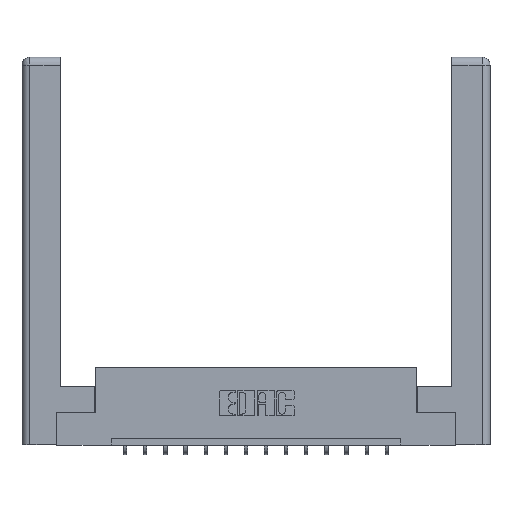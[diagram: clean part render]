
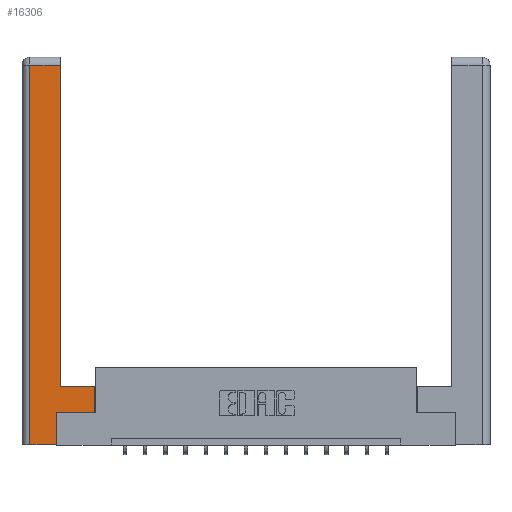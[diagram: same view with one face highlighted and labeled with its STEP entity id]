
A CAD part, top view. The second image highlights one B-rep face of the part: STEP entity #16306.
In plain terms, the highlighted planar face has unit normal (0, 0, 1).
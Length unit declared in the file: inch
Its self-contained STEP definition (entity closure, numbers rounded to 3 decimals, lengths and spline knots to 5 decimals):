
#33 = VECTOR ( 'NONE', #9233, 39.37008 ) ;
#392 = VERTEX_POINT ( 'NONE', #15237 ) ;
#905 = CARTESIAN_POINT ( 'NONE',  ( 0.265, 0.245, 0. ) ) ;
#1146 = LINE ( 'NONE', #4113, #2574 ) ;
#1527 = VERTEX_POINT ( 'NONE', #14548 ) ;
#2090 = CARTESIAN_POINT ( 'NONE',  ( 0.0615, 2.94, 0. ) ) ;
#2414 = CARTESIAN_POINT ( 'NONE',  ( 0.565, 0.45, 0. ) ) ;
#2574 = VECTOR ( 'NONE', #15525, 39.37008 ) ;
#2589 = DIRECTION ( 'NONE',  ( -1., 0., 0. ) ) ;
#2604 = VECTOR ( 'NONE', #15812, 39.37008 ) ;
#2819 = ORIENTED_EDGE ( 'NONE', *, *, #16593, .T. ) ;
#3337 = CARTESIAN_POINT ( 'NONE',  ( 0.565, 0.45, 0. ) ) ;
#3830 = CARTESIAN_POINT ( 'NONE',  ( 0.565, 0.245, 0. ) ) ;
#3939 = DIRECTION ( 'NONE',  ( 1., 0., 0. ) ) ;
#4113 = CARTESIAN_POINT ( 'NONE',  ( 0.0615, 0., 0. ) ) ;
#4242 = CARTESIAN_POINT ( 'NONE',  ( 0.295, 3., 0. ) ) ;
#4461 = VERTEX_POINT ( 'NONE', #2090 ) ;
#4954 = VERTEX_POINT ( 'NONE', #13123 ) ;
#5233 = LINE ( 'NONE', #2414, #7033 ) ;
#5357 = VECTOR ( 'NONE', #7497, 39.37008 ) ;
#5381 = EDGE_CURVE ( 'NONE', #392, #14275, #13060, .T. ) ;
#6147 = EDGE_CURVE ( 'NONE', #7818, #11671, #10586, .T. ) ;
#6274 = CARTESIAN_POINT ( 'NONE',  ( 0.295, 0.45, 0. ) ) ;
#6314 = CARTESIAN_POINT ( 'NONE',  ( 0.0615, 2.94, 0. ) ) ;
#6333 = DIRECTION ( 'NONE',  ( 0., 1., 0. ) ) ;
#7033 = VECTOR ( 'NONE', #6333, 39.37008 ) ;
#7497 = DIRECTION ( 'NONE',  ( 0., 1., 0. ) ) ;
#7818 = VERTEX_POINT ( 'NONE', #3337 ) ;
#8476 = LINE ( 'NONE', #15450, #15582 ) ;
#9026 = DIRECTION ( 'NONE',  ( 0., 0., -1. ) ) ;
#9233 = DIRECTION ( 'NONE',  ( -1., 0., 0. ) ) ;
#9713 = CARTESIAN_POINT ( 'NONE',  ( 0.265, 0., 0. ) ) ;
#9742 = ORIENTED_EDGE ( 'NONE', *, *, #6147, .T. ) ;
#9832 = LINE ( 'NONE', #9713, #12288 ) ;
#9867 = ORIENTED_EDGE ( 'NONE', *, *, #14572, .T. ) ;
#10187 = VECTOR ( 'NONE', #10888, 39.37008 ) ;
#10586 = LINE ( 'NONE', #15915, #33 ) ;
#10695 = EDGE_CURVE ( 'NONE', #4954, #4461, #14246, .T. ) ;
#10888 = DIRECTION ( 'NONE',  ( -1., 0., 0. ) ) ;
#11099 = FACE_OUTER_BOUND ( 'NONE', #14337, .T. ) ;
#11671 = VERTEX_POINT ( 'NONE', #6274 ) ;
#11720 = DIRECTION ( 'NONE',  ( 1., 0., 0. ) ) ;
#12142 = ORIENTED_EDGE ( 'NONE', *, *, #16000, .T. ) ;
#12288 = VECTOR ( 'NONE', #11720, 39.37008 ) ;
#12792 = VERTEX_POINT ( 'NONE', #3830 ) ;
#12911 = PLANE ( 'NONE',  #12947 ) ;
#12947 = AXIS2_PLACEMENT_3D ( 'NONE', #16766, #9026, #2589 ) ;
#12950 = LINE ( 'NONE', #4242, #2604 ) ;
#13060 = LINE ( 'NONE', #905, #5357 ) ;
#13123 = CARTESIAN_POINT ( 'NONE',  ( 0.295, 2.94, 0. ) ) ;
#13179 = EDGE_CURVE ( 'NONE', #14275, #12792, #8476, .T. ) ;
#13532 = ORIENTED_EDGE ( 'NONE', *, *, #13179, .T. ) ;
#13865 = EDGE_CURVE ( 'NONE', #12792, #7818, #5233, .T. ) ;
#14082 = ORIENTED_EDGE ( 'NONE', *, *, #10695, .T. ) ;
#14246 = LINE ( 'NONE', #6314, #10187 ) ;
#14275 = VERTEX_POINT ( 'NONE', #14389 ) ;
#14337 = EDGE_LOOP ( 'NONE', ( #12142, #14082, #2819, #9867, #14625, #13532, #15276, #9742 ) ) ;
#14389 = CARTESIAN_POINT ( 'NONE',  ( 0.265, 0.245, 0. ) ) ;
#14548 = CARTESIAN_POINT ( 'NONE',  ( 0.0615, 0., 0. ) ) ;
#14572 = EDGE_CURVE ( 'NONE', #1527, #392, #9832, .T. ) ;
#14625 = ORIENTED_EDGE ( 'NONE', *, *, #5381, .T. ) ;
#15237 = CARTESIAN_POINT ( 'NONE',  ( 0.265, 0., 0. ) ) ;
#15276 = ORIENTED_EDGE ( 'NONE', *, *, #13865, .T. ) ;
#15450 = CARTESIAN_POINT ( 'NONE',  ( 0.565, 0.245, 0. ) ) ;
#15525 = DIRECTION ( 'NONE',  ( 0., -1., 0. ) ) ;
#15582 = VECTOR ( 'NONE', #3939, 39.37008 ) ;
#15812 = DIRECTION ( 'NONE',  ( 0., 1., 0. ) ) ;
#15915 = CARTESIAN_POINT ( 'NONE',  ( 0.295, 0.45, 0. ) ) ;
#16000 = EDGE_CURVE ( 'NONE', #11671, #4954, #12950, .T. ) ;
#16306 = ADVANCED_FACE ( 'NONE', ( #11099 ), #12911, .F. ) ;
#16593 = EDGE_CURVE ( 'NONE', #4461, #1527, #1146, .T. ) ;
#16766 = CARTESIAN_POINT ( 'NONE',  ( 0., 0., 0. ) ) ;
